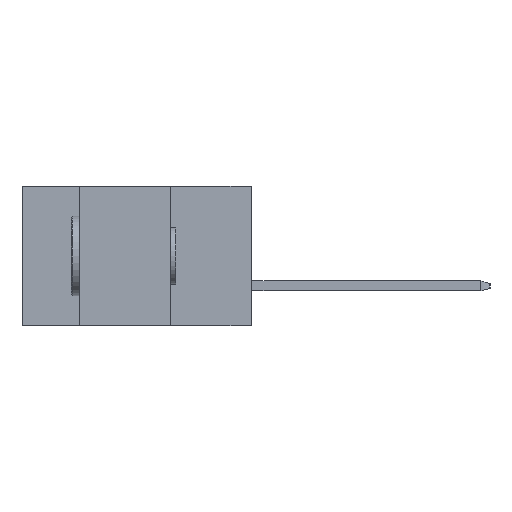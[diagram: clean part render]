
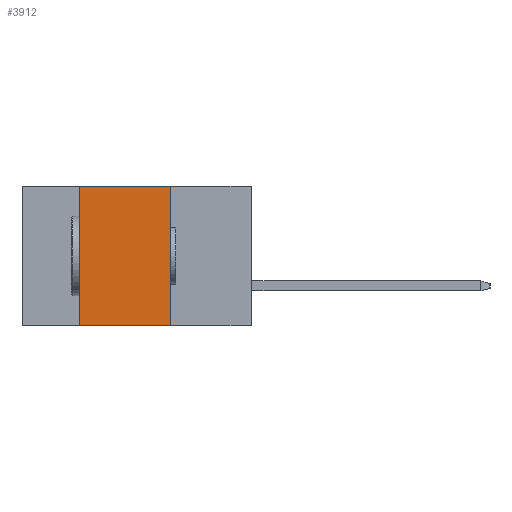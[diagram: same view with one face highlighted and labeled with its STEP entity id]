
A CAD part, left-side view. The second image highlights one B-rep face of the part: STEP entity #3912.
In plain terms, the highlighted planar face has unit normal (-1, 0, 0).
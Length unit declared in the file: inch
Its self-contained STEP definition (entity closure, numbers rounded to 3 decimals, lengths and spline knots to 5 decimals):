
#234 = EDGE_CURVE ( 'NONE', #1122, #8086, #5755, .T. ) ;
#659 = CARTESIAN_POINT ( 'NONE',  ( 0., 0.72, 0. ) ) ;
#1122 = VERTEX_POINT ( 'NONE', #10267 ) ;
#1475 = DIRECTION ( 'NONE',  ( 1., 0., 0. ) ) ;
#1511 = ORIENTED_EDGE ( 'NONE', *, *, #234, .F. ) ;
#2310 = DIRECTION ( 'NONE',  ( 0., 0., -1. ) ) ;
#2531 = AXIS2_PLACEMENT_3D ( 'NONE', #659, #1475, #2310 ) ;
#3072 = LINE ( 'NONE', #7432, #8231 ) ;
#3138 = EDGE_CURVE ( 'NONE', #5078, #1122, #9968, .T. ) ;
#3201 = DIRECTION ( 'NONE',  ( 0., -1., 0. ) ) ;
#3868 = VECTOR ( 'NONE', #10803, 39.37008 ) ;
#3912 = ADVANCED_FACE ( 'NONE', ( #9892 ), #4947, .F. ) ;
#4100 = CARTESIAN_POINT ( 'NONE',  ( 0., 0.72, 0. ) ) ;
#4199 = VERTEX_POINT ( 'NONE', #7971 ) ;
#4927 = EDGE_LOOP ( 'NONE', ( #1511, #6773, #10048, #9988 ) ) ;
#4947 = PLANE ( 'NONE',  #2531 ) ;
#5078 = VERTEX_POINT ( 'NONE', #5913 ) ;
#5724 = DIRECTION ( 'NONE',  ( 0., 0., 1. ) ) ;
#5755 = LINE ( 'NONE', #9756, #10669 ) ;
#5913 = CARTESIAN_POINT ( 'NONE',  ( 0., 0.54, 0. ) ) ;
#6546 = EDGE_CURVE ( 'NONE', #4199, #8086, #8369, .T. ) ;
#6634 = DIRECTION ( 'NONE',  ( 0., 0., -1. ) ) ;
#6773 = ORIENTED_EDGE ( 'NONE', *, *, #3138, .F. ) ;
#6980 = EDGE_CURVE ( 'NONE', #4199, #5078, #3072, .T. ) ;
#7432 = CARTESIAN_POINT ( 'NONE',  ( 0., 0.54, -0.437 ) ) ;
#7971 = CARTESIAN_POINT ( 'NONE',  ( 0., 0.54, -0.437 ) ) ;
#8086 = VERTEX_POINT ( 'NONE', #9529 ) ;
#8231 = VECTOR ( 'NONE', #5724, 39.37008 ) ;
#8369 = LINE ( 'NONE', #9845, #10497 ) ;
#9529 = CARTESIAN_POINT ( 'NONE',  ( 0., 0.254, -0.437 ) ) ;
#9756 = CARTESIAN_POINT ( 'NONE',  ( 0., 0.254, -0.437 ) ) ;
#9845 = CARTESIAN_POINT ( 'NONE',  ( 0., 0.72, -0.437 ) ) ;
#9892 = FACE_OUTER_BOUND ( 'NONE', #4927, .T. ) ;
#9968 = LINE ( 'NONE', #4100, #3868 ) ;
#9988 = ORIENTED_EDGE ( 'NONE', *, *, #6546, .T. ) ;
#10048 = ORIENTED_EDGE ( 'NONE', *, *, #6980, .F. ) ;
#10267 = CARTESIAN_POINT ( 'NONE',  ( 0., 0.254, 0. ) ) ;
#10497 = VECTOR ( 'NONE', #3201, 39.37008 ) ;
#10669 = VECTOR ( 'NONE', #6634, 39.37008 ) ;
#10803 = DIRECTION ( 'NONE',  ( 0., -1., 0. ) ) ;
